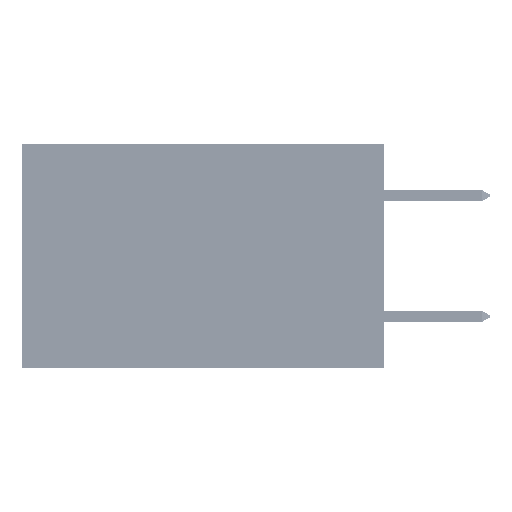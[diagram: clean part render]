
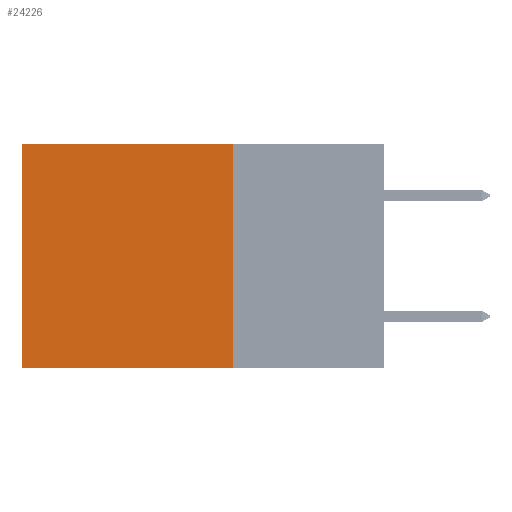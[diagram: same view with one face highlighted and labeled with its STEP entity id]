
A CAD part, left-side view. The second image highlights one B-rep face of the part: STEP entity #24226.
In plain terms, the highlighted planar face has unit normal (-1, 0, 0).
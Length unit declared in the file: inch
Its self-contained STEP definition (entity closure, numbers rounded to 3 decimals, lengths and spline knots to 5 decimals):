
#2877 = CARTESIAN_POINT ( 'NONE',  ( 0.2875, 0.6, 0. ) ) ;
#3294 = VERTEX_POINT ( 'NONE', #5697 ) ;
#3869 = PLANE ( 'NONE',  #4254 ) ;
#4046 = DIRECTION ( 'NONE',  ( 0., 0., -1. ) ) ;
#4254 = AXIS2_PLACEMENT_3D ( 'NONE', #22838, #26799, #4046 ) ;
#5697 = CARTESIAN_POINT ( 'NONE',  ( 0.2875, 0.6, -0.37 ) ) ;
#6577 = ORIENTED_EDGE ( 'NONE', *, *, #22024, .T. ) ;
#7193 = VERTEX_POINT ( 'NONE', #42383 ) ;
#11410 = ORIENTED_EDGE ( 'NONE', *, *, #32914, .F. ) ;
#11513 = VERTEX_POINT ( 'NONE', #40581 ) ;
#11671 = VERTEX_POINT ( 'NONE', #22750 ) ;
#12382 = DIRECTION ( 'NONE',  ( 0., 0., -1. ) ) ;
#13914 = CARTESIAN_POINT ( 'NONE',  ( 0.2875, 0.25, 0. ) ) ;
#14455 = LINE ( 'NONE', #13914, #32127 ) ;
#15104 = VECTOR ( 'NONE', #25682, 39.37008 ) ;
#15425 = ORIENTED_EDGE ( 'NONE', *, *, #36676, .F. ) ;
#17739 = DIRECTION ( 'NONE',  ( 0., 1., 0. ) ) ;
#20356 = DIRECTION ( 'NONE',  ( 0., 1., 0. ) ) ;
#20893 = ORIENTED_EDGE ( 'NONE', *, *, #39954, .T. ) ;
#21163 = LINE ( 'NONE', #31158, #29992 ) ;
#22024 = EDGE_CURVE ( 'NONE', #11513, #11671, #14455, .T. ) ;
#22750 = CARTESIAN_POINT ( 'NONE',  ( 0.2875, 0.6, 0. ) ) ;
#22838 = CARTESIAN_POINT ( 'NONE',  ( 0.2875, 0.25, 0. ) ) ;
#24226 = ADVANCED_FACE ( 'NONE', ( #26635 ), #3869, .F. ) ;
#25156 = LINE ( 'NONE', #2877, #15104 ) ;
#25682 = DIRECTION ( 'NONE',  ( 0., 0., -1. ) ) ;
#25870 = EDGE_LOOP ( 'NONE', ( #20893, #15425, #11410, #6577 ) ) ;
#26635 = FACE_OUTER_BOUND ( 'NONE', #25870, .T. ) ;
#26799 = DIRECTION ( 'NONE',  ( 1., 0., 0. ) ) ;
#29011 = VECTOR ( 'NONE', #20356, 39.37008 ) ;
#29992 = VECTOR ( 'NONE', #12382, 39.37008 ) ;
#31158 = CARTESIAN_POINT ( 'NONE',  ( 0.2875, 0.25, 0. ) ) ;
#31546 = CARTESIAN_POINT ( 'NONE',  ( 0.2875, 0.25, -0.37 ) ) ;
#32127 = VECTOR ( 'NONE', #17739, 39.37008 ) ;
#32914 = EDGE_CURVE ( 'NONE', #11513, #7193, #21163, .T. ) ;
#36676 = EDGE_CURVE ( 'NONE', #7193, #3294, #45649, .T. ) ;
#39954 = EDGE_CURVE ( 'NONE', #11671, #3294, #25156, .T. ) ;
#40581 = CARTESIAN_POINT ( 'NONE',  ( 0.2875, 0.25, 0. ) ) ;
#42383 = CARTESIAN_POINT ( 'NONE',  ( 0.2875, 0.25, -0.37 ) ) ;
#45649 = LINE ( 'NONE', #31546, #29011 ) ;
